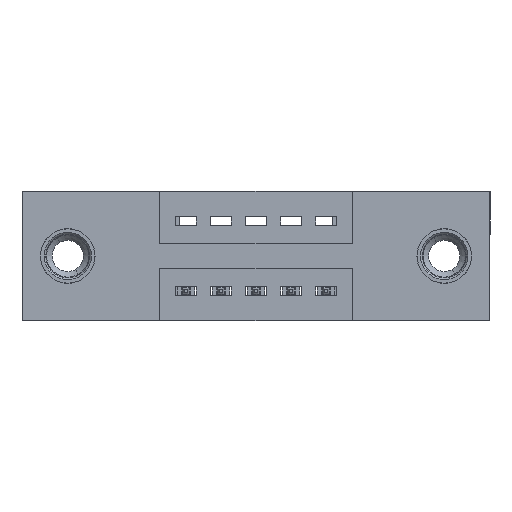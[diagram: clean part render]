
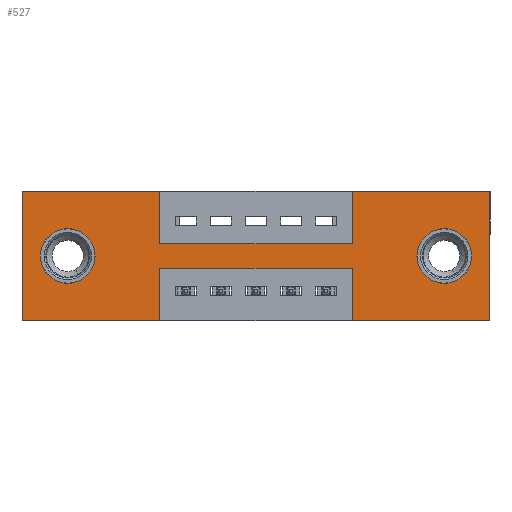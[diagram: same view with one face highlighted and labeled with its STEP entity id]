
A CAD part, front view. The second image highlights one B-rep face of the part: STEP entity #527.
In plain terms, the highlighted planar face has unit normal (0, -1, 0).
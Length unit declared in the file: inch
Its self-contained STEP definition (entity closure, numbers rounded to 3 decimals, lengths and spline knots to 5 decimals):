
#37 = EDGE_LOOP ( 'NONE', ( #318, #10411 ) ) ;
#212 = ORIENTED_EDGE ( 'NONE', *, *, #13078, .F. ) ;
#266 = VECTOR ( 'NONE', #6261, 39.37008 ) ;
#318 = ORIENTED_EDGE ( 'NONE', *, *, #13114, .T. ) ;
#418 = EDGE_CURVE ( 'NONE', #6302, #3063, #12730, .T. ) ;
#422 = CARTESIAN_POINT ( 'NONE',  ( 0.3925, 0., 0. ) ) ;
#527 = ADVANCED_FACE ( 'NONE', ( #6186, #7314, #5047 ), #9248, .T. ) ;
#566 = EDGE_CURVE ( 'NONE', #12111, #10041, #11074, .T. ) ;
#912 = EDGE_CURVE ( 'NONE', #10041, #12111, #4048, .T. ) ;
#997 = LINE ( 'NONE', #2591, #2817 ) ;
#1264 = CARTESIAN_POINT ( 'NONE',  ( 1.205, 0., -0.185 ) ) ;
#1446 = CARTESIAN_POINT ( 'NONE',  ( 0.13, 0., -0.185 ) ) ;
#1467 = CARTESIAN_POINT ( 'NONE',  ( 0.9425, 0., -0.37 ) ) ;
#1514 = CARTESIAN_POINT ( 'NONE',  ( 0.13, 0., -0.107 ) ) ;
#1561 = AXIS2_PLACEMENT_3D ( 'NONE', #7630, #2473, #8681 ) ;
#1604 = EDGE_CURVE ( 'NONE', #8934, #4786, #4197, .T. ) ;
#1845 = VERTEX_POINT ( 'NONE', #11850 ) ;
#2275 = DIRECTION ( 'NONE',  ( 0., 0., -1. ) ) ;
#2326 = LINE ( 'NONE', #2559, #8847 ) ;
#2331 = EDGE_CURVE ( 'NONE', #11336, #1845, #11646, .T. ) ;
#2373 = CARTESIAN_POINT ( 'NONE',  ( 0.3925, 0., -0.37 ) ) ;
#2473 = DIRECTION ( 'NONE',  ( 0., 1., 0. ) ) ;
#2517 = VERTEX_POINT ( 'NONE', #6888 ) ;
#2559 = CARTESIAN_POINT ( 'NONE',  ( 0., 0., 0. ) ) ;
#2591 = CARTESIAN_POINT ( 'NONE',  ( 0., 0., -0.37 ) ) ;
#2817 = VECTOR ( 'NONE', #10015, 39.37008 ) ;
#2939 = CARTESIAN_POINT ( 'NONE',  ( 0.9425, 0., -0.22 ) ) ;
#2955 = CARTESIAN_POINT ( 'NONE',  ( 0.3925, 0., -0.15 ) ) ;
#3063 = VERTEX_POINT ( 'NONE', #9769 ) ;
#3131 = VECTOR ( 'NONE', #12802, 39.37008 ) ;
#3193 = ORIENTED_EDGE ( 'NONE', *, *, #6467, .F. ) ;
#3276 = VECTOR ( 'NONE', #8485, 39.37008 ) ;
#3357 = VERTEX_POINT ( 'NONE', #6050 ) ;
#3385 = EDGE_LOOP ( 'NONE', ( #4113, #10860 ) ) ;
#3536 = EDGE_CURVE ( 'NONE', #10070, #8934, #997, .T. ) ;
#3629 = ORIENTED_EDGE ( 'NONE', *, *, #13474, .F. ) ;
#3672 = EDGE_CURVE ( 'NONE', #1845, #10070, #4273, .T. ) ;
#3744 = CARTESIAN_POINT ( 'NONE',  ( 1.205, 0., -0.263 ) ) ;
#3791 = CARTESIAN_POINT ( 'NONE',  ( 0.9425, 0., 0. ) ) ;
#3853 = VERTEX_POINT ( 'NONE', #13252 ) ;
#4048 = CIRCLE ( 'NONE', #5705, 0.078 ) ;
#4113 = ORIENTED_EDGE ( 'NONE', *, *, #566, .T. ) ;
#4197 = LINE ( 'NONE', #1467, #13200 ) ;
#4273 = LINE ( 'NONE', #8359, #10796 ) ;
#4468 = DIRECTION ( 'NONE',  ( 1., 0., 0. ) ) ;
#4615 = ORIENTED_EDGE ( 'NONE', *, *, #3536, .F. ) ;
#4786 = VERTEX_POINT ( 'NONE', #2939 ) ;
#4803 = ORIENTED_EDGE ( 'NONE', *, *, #6510, .F. ) ;
#4975 = VECTOR ( 'NONE', #11734, 39.37008 ) ;
#5047 = FACE_OUTER_BOUND ( 'NONE', #10331, .T. ) ;
#5086 = LINE ( 'NONE', #8781, #3131 ) ;
#5224 = CARTESIAN_POINT ( 'NONE',  ( 0., 0., -0.37 ) ) ;
#5233 = LINE ( 'NONE', #8575, #3276 ) ;
#5258 = DIRECTION ( 'NONE',  ( 0., 0., -1. ) ) ;
#5305 = LINE ( 'NONE', #2373, #4975 ) ;
#5311 = VERTEX_POINT ( 'NONE', #1514 ) ;
#5346 = CARTESIAN_POINT ( 'NONE',  ( 0.9425, 0., 0. ) ) ;
#5603 = ORIENTED_EDGE ( 'NONE', *, *, #7793, .F. ) ;
#5672 = LINE ( 'NONE', #12482, #11886 ) ;
#5705 = AXIS2_PLACEMENT_3D ( 'NONE', #9315, #10351, #12462 ) ;
#5773 = VECTOR ( 'NONE', #13510, 39.37008 ) ;
#6050 = CARTESIAN_POINT ( 'NONE',  ( 0., 0., -0.37 ) ) ;
#6186 = FACE_BOUND ( 'NONE', #3385, .T. ) ;
#6261 = DIRECTION ( 'NONE',  ( 0., 0., 1. ) ) ;
#6294 = LINE ( 'NONE', #5346, #12851 ) ;
#6302 = VERTEX_POINT ( 'NONE', #10822 ) ;
#6467 = EDGE_CURVE ( 'NONE', #8404, #6302, #5672, .T. ) ;
#6510 = EDGE_CURVE ( 'NONE', #3357, #7645, #11059, .T. ) ;
#6558 = DIRECTION ( 'NONE',  ( 0., 1., 0. ) ) ;
#6857 = EDGE_CURVE ( 'NONE', #3853, #5311, #7124, .T. ) ;
#6888 = CARTESIAN_POINT ( 'NONE',  ( 0.3925, 0., -0.37 ) ) ;
#7124 = CIRCLE ( 'NONE', #11175, 0.078 ) ;
#7314 = FACE_BOUND ( 'NONE', #37, .T. ) ;
#7630 = CARTESIAN_POINT ( 'NONE',  ( 0.13, 0., -0.185 ) ) ;
#7645 = VERTEX_POINT ( 'NONE', #9069 ) ;
#7793 = EDGE_CURVE ( 'NONE', #3063, #11336, #6294, .T. ) ;
#7890 = CARTESIAN_POINT ( 'NONE',  ( 1.205, 0., -0.107 ) ) ;
#8325 = CARTESIAN_POINT ( 'NONE',  ( 0., 0., 0. ) ) ;
#8334 = DIRECTION ( 'NONE',  ( 0., -1., 0. ) ) ;
#8359 = CARTESIAN_POINT ( 'NONE',  ( 1.335, 0., 0. ) ) ;
#8404 = VERTEX_POINT ( 'NONE', #422 ) ;
#8485 = DIRECTION ( 'NONE',  ( -1., 0., 0. ) ) ;
#8526 = DIRECTION ( 'NONE',  ( 0., 1., 0. ) ) ;
#8575 = CARTESIAN_POINT ( 'NONE',  ( 0.3925, 0., -0.22 ) ) ;
#8632 = DIRECTION ( 'NONE',  ( 0., 0., -1. ) ) ;
#8681 = DIRECTION ( 'NONE',  ( 0., 0., 1. ) ) ;
#8761 = ORIENTED_EDGE ( 'NONE', *, *, #8955, .F. ) ;
#8763 = DIRECTION ( 'NONE',  ( 0., 0., 1. ) ) ;
#8781 = CARTESIAN_POINT ( 'NONE',  ( 0., 0., -0.37 ) ) ;
#8847 = VECTOR ( 'NONE', #4468, 39.37008 ) ;
#8934 = VERTEX_POINT ( 'NONE', #11774 ) ;
#8955 = EDGE_CURVE ( 'NONE', #7645, #8404, #2326, .T. ) ;
#9069 = CARTESIAN_POINT ( 'NONE',  ( 0., 0., 0. ) ) ;
#9075 = ORIENTED_EDGE ( 'NONE', *, *, #10424, .F. ) ;
#9248 = PLANE ( 'NONE',  #12245 ) ;
#9315 = CARTESIAN_POINT ( 'NONE',  ( 1.205, 0., -0.185 ) ) ;
#9334 = ORIENTED_EDGE ( 'NONE', *, *, #1604, .F. ) ;
#9441 = CARTESIAN_POINT ( 'NONE',  ( 0.3925, 0., -0.22 ) ) ;
#9769 = CARTESIAN_POINT ( 'NONE',  ( 0.9425, 0., -0.15 ) ) ;
#9784 = VECTOR ( 'NONE', #10244, 39.37008 ) ;
#9786 = DIRECTION ( 'NONE',  ( 0., 0., 1. ) ) ;
#10015 = DIRECTION ( 'NONE',  ( -1., 0., 0. ) ) ;
#10041 = VERTEX_POINT ( 'NONE', #3744 ) ;
#10070 = VERTEX_POINT ( 'NONE', #13175 ) ;
#10244 = DIRECTION ( 'NONE',  ( 1., 0., 0. ) ) ;
#10289 = CIRCLE ( 'NONE', #1561, 0.078 ) ;
#10331 = EDGE_LOOP ( 'NONE', ( #9075, #3629, #9334, #4615, #12442, #12634, #5603, #11538, #3193, #8761, #4803, #212 ) ) ;
#10351 = DIRECTION ( 'NONE',  ( 0., 1., 0. ) ) ;
#10411 = ORIENTED_EDGE ( 'NONE', *, *, #6857, .T. ) ;
#10424 = EDGE_CURVE ( 'NONE', #11008, #2517, #5305, .T. ) ;
#10796 = VECTOR ( 'NONE', #8632, 39.37008 ) ;
#10822 = CARTESIAN_POINT ( 'NONE',  ( 0.3925, 0., -0.15 ) ) ;
#10860 = ORIENTED_EDGE ( 'NONE', *, *, #912, .T. ) ;
#11008 = VERTEX_POINT ( 'NONE', #9441 ) ;
#11059 = LINE ( 'NONE', #8325, #266 ) ;
#11074 = CIRCLE ( 'NONE', #11285, 0.078 ) ;
#11175 = AXIS2_PLACEMENT_3D ( 'NONE', #1446, #6558, #8763 ) ;
#11285 = AXIS2_PLACEMENT_3D ( 'NONE', #1264, #8526, #2275 ) ;
#11336 = VERTEX_POINT ( 'NONE', #3791 ) ;
#11538 = ORIENTED_EDGE ( 'NONE', *, *, #418, .F. ) ;
#11646 = LINE ( 'NONE', #12354, #5773 ) ;
#11731 = DIRECTION ( 'NONE',  ( 0., 0., 1. ) ) ;
#11734 = DIRECTION ( 'NONE',  ( 0., 0., -1. ) ) ;
#11774 = CARTESIAN_POINT ( 'NONE',  ( 0.9425, 0., -0.37 ) ) ;
#11850 = CARTESIAN_POINT ( 'NONE',  ( 1.335, 0., 0. ) ) ;
#11886 = VECTOR ( 'NONE', #5258, 39.37008 ) ;
#12111 = VERTEX_POINT ( 'NONE', #7890 ) ;
#12245 = AXIS2_PLACEMENT_3D ( 'NONE', #5224, #8334, #13598 ) ;
#12354 = CARTESIAN_POINT ( 'NONE',  ( 0., 0., 0. ) ) ;
#12442 = ORIENTED_EDGE ( 'NONE', *, *, #3672, .F. ) ;
#12462 = DIRECTION ( 'NONE',  ( 0., 0., -1. ) ) ;
#12482 = CARTESIAN_POINT ( 'NONE',  ( 0.3925, 0., 0. ) ) ;
#12634 = ORIENTED_EDGE ( 'NONE', *, *, #2331, .F. ) ;
#12730 = LINE ( 'NONE', #2955, #9784 ) ;
#12802 = DIRECTION ( 'NONE',  ( -1., 0., 0. ) ) ;
#12851 = VECTOR ( 'NONE', #11731, 39.37008 ) ;
#13078 = EDGE_CURVE ( 'NONE', #2517, #3357, #5086, .T. ) ;
#13114 = EDGE_CURVE ( 'NONE', #5311, #3853, #10289, .T. ) ;
#13175 = CARTESIAN_POINT ( 'NONE',  ( 1.335, 0., -0.37 ) ) ;
#13200 = VECTOR ( 'NONE', #9786, 39.37008 ) ;
#13252 = CARTESIAN_POINT ( 'NONE',  ( 0.13, 0., -0.263 ) ) ;
#13474 = EDGE_CURVE ( 'NONE', #4786, #11008, #5233, .T. ) ;
#13510 = DIRECTION ( 'NONE',  ( 1., 0., 0. ) ) ;
#13598 = DIRECTION ( 'NONE',  ( 0., 0., -1. ) ) ;
